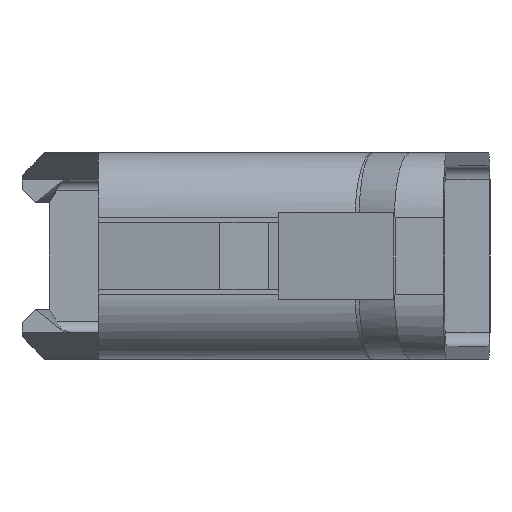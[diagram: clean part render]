
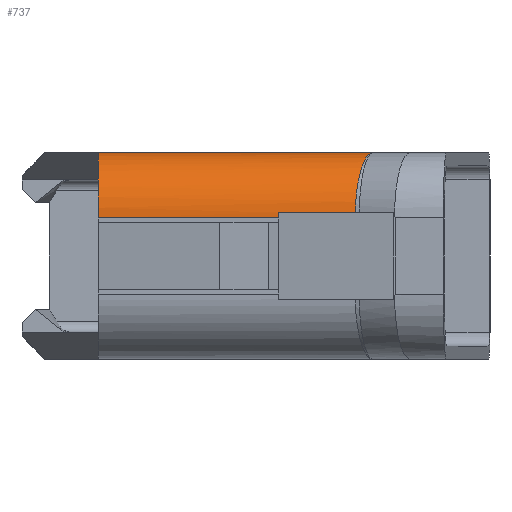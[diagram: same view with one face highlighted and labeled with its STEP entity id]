
A CAD part, left-side view. The second image highlights one B-rep face of the part: STEP entity #737.
In plain terms, the highlighted cylindrical face has radius 6 mm (diameter 12 mm), a partial arc.
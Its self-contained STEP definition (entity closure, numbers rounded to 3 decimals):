
#217 = VERTEX_POINT ( 'NONE', #3966 ) ;
#241 = VERTEX_POINT ( 'NONE', #4013 ) ;
#262 = EDGE_CURVE ( 'NONE', #217, #241, #3999, .T. ) ;
#668 = EDGE_CURVE ( 'NONE', #684, #685, #4780, .T. ) ;
#684 = VERTEX_POINT ( 'NONE', #4790 ) ;
#685 = VERTEX_POINT ( 'NONE', #4776 ) ;
#712 = ORIENTED_EDGE ( 'NONE', *, *, #262, .F. ) ;
#716 = EDGE_LOOP ( 'NONE', ( #738, #722, #712, #717, #728, #751 ) ) ;
#717 = ORIENTED_EDGE ( 'NONE', *, *, #736, .F. ) ;
#721 = EDGE_CURVE ( 'NONE', #684, #739, #4863, .T. ) ;
#722 = ORIENTED_EDGE ( 'NONE', *, *, #735, .T. ) ;
#728 = ORIENTED_EDGE ( 'NONE', *, *, #668, .F. ) ;
#731 = VERTEX_POINT ( 'NONE', #4905 ) ;
#734 = EDGE_CURVE ( 'NONE', #739, #731, #4903, .T. ) ;
#735 = EDGE_CURVE ( 'NONE', #731, #241, #4919, .T. ) ;
#736 = EDGE_CURVE ( 'NONE', #685, #217, #4910, .T. ) ;
#737 = ADVANCED_FACE ( 'NONE', ( #4872 ), #4898, .T. ) ;
#738 = ORIENTED_EDGE ( 'NONE', *, *, #734, .T. ) ;
#739 = VERTEX_POINT ( 'NONE', #4950 ) ;
#751 = ORIENTED_EDGE ( 'NONE', *, *, #721, .T. ) ;
#3966 = CARTESIAN_POINT ( 'NONE',  ( 6.007, 0., 9.5 ) ) ;
#3999 = LINE ( 'NONE', #4047, #4046 ) ;
#4013 = CARTESIAN_POINT ( 'NONE',  ( 4.821, -25.309, 9.5 ) ) ;
#4045 = DIRECTION ( 'NONE',  ( -0.047, -0.999, 0. ) ) ;
#4046 = VECTOR ( 'NONE', #4045, 1000. ) ;
#4047 = CARTESIAN_POINT ( 'NONE',  ( 4.875, -24.155, 9.5 ) ) ;
#4776 = CARTESIAN_POINT ( 'NONE',  ( 0., 0., 3.5 ) ) ;
#4777 = DIRECTION ( 'NONE',  ( 0.047, 0.999, 0. ) ) ;
#4778 = VECTOR ( 'NONE', #4777, 1000. ) ;
#4779 = CARTESIAN_POINT ( 'NONE',  ( 0., 0., 3.5 ) ) ;
#4780 = LINE ( 'NONE', #4779, #4778 ) ;
#4790 = CARTESIAN_POINT ( 'NONE',  ( -0.777, -16.582, 3.5 ) ) ;
#4862 = CARTESIAN_POINT ( 'NONE',  ( -0.777, -16.582, 3.5 ) ) ;
#4863 =( BOUNDED_CURVE ( )  B_SPLINE_CURVE ( 3, ( #4862, #4891, #4890, #4889 ),
 .UNSPECIFIED., .F., .T. ) 
 B_SPLINE_CURVE_WITH_KNOTS ( ( 4, 4 ),
 ( 3.142, 3.225 ),
 .UNSPECIFIED. ) 
 CURVE ( )  GEOMETRIC_REPRESENTATION_ITEM ( )  RATIONAL_B_SPLINE_CURVE ( ( 1., 0.999, 0.999, 1. ) ) 
 REPRESENTATION_ITEM ( '' )  );
#4872 = FACE_OUTER_BOUND ( 'NONE', #716, .T. ) ;
#4889 = CARTESIAN_POINT ( 'NONE',  ( -0.756, -16.582, 4. ) ) ;
#4890 = CARTESIAN_POINT ( 'NONE',  ( -0.77, -16.582, 3.834 ) ) ;
#4891 = CARTESIAN_POINT ( 'NONE',  ( -0.777, -16.582, 3.667 ) ) ;
#4898 = CYLINDRICAL_SURFACE ( 'NONE', #4920, 6. ) ;
#4903 = LINE ( 'NONE', #4925, #4924 ) ;
#4905 = CARTESIAN_POINT ( 'NONE',  ( -1.089, -23.688, 4. ) ) ;
#4906 = CARTESIAN_POINT ( 'NONE',  ( 6.007, 0., 9.5 ) ) ;
#4907 = CARTESIAN_POINT ( 'NONE',  ( 2.488, 0., 9.5 ) ) ;
#4908 = CARTESIAN_POINT ( 'NONE',  ( 0., 0., 7.015 ) ) ;
#4909 = CARTESIAN_POINT ( 'NONE',  ( 0., 0., 3.5 ) ) ;
#4910 =( BOUNDED_CURVE ( )  B_SPLINE_CURVE ( 3, ( #4909, #4908, #4907, #4906 ),
 .UNSPECIFIED., .F., .F. ) 
 B_SPLINE_CURVE_WITH_KNOTS ( ( 4, 4 ),
 ( 3.142, 4.712 ),
 .UNSPECIFIED. ) 
 CURVE ( )  GEOMETRIC_REPRESENTATION_ITEM ( )  RATIONAL_B_SPLINE_CURVE ( ( 1., 0.805, 0.805, 1. ) ) 
 REPRESENTATION_ITEM ( '' )  );
#4911 = DIRECTION ( 'NONE',  ( -0.999, 0.047, 0. ) ) ;
#4914 = CARTESIAN_POINT ( 'NONE',  ( 4.821, -25.309, 9.5 ) ) ;
#4915 = CARTESIAN_POINT ( 'NONE',  ( 1.573, -24.418, 9.5 ) ) ;
#4916 = CARTESIAN_POINT ( 'NONE',  ( -0.818, -23.762, 7.275 ) ) ;
#4917 = CARTESIAN_POINT ( 'NONE',  ( -1.089, -23.688, 4. ) ) ;
#4918 = DIRECTION ( 'NONE',  ( 0.047, 0.999, 0. ) ) ;
#4919 =( BOUNDED_CURVE ( )  B_SPLINE_CURVE ( 3, ( #4917, #4916, #4915, #4914 ),
 .UNSPECIFIED., .F., .F. ) 
 B_SPLINE_CURVE_WITH_KNOTS ( ( 4, 4 ),
 ( 3.225, 4.712 ),
 .UNSPECIFIED. ) 
 CURVE ( )  GEOMETRIC_REPRESENTATION_ITEM ( )  RATIONAL_B_SPLINE_CURVE ( ( 1., 0.824, 0.824, 1. ) ) 
 REPRESENTATION_ITEM ( '' )  );
#4920 = AXIS2_PLACEMENT_3D ( 'NONE', #4921, #4918, #4911 ) ;
#4921 = CARTESIAN_POINT ( 'NONE',  ( 4.501, -32.146, 3.5 ) ) ;
#4923 = DIRECTION ( 'NONE',  ( -0.047, -0.999, 0. ) ) ;
#4924 = VECTOR ( 'NONE', #4923, 1000. ) ;
#4925 = CARTESIAN_POINT ( 'NONE',  ( -1.472, -31.866, 4. ) ) ;
#4950 = CARTESIAN_POINT ( 'NONE',  ( -0.756, -16.582, 4. ) ) ;
